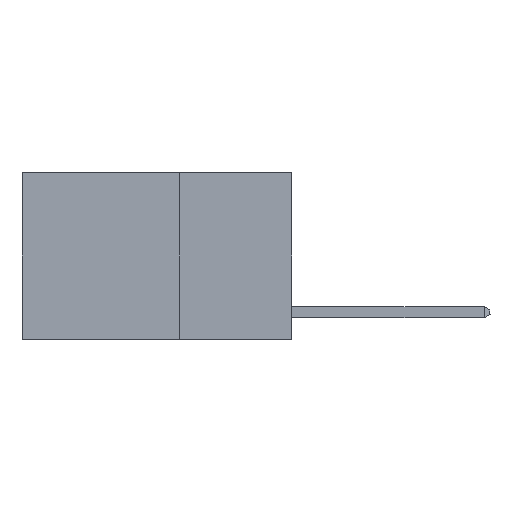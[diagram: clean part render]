
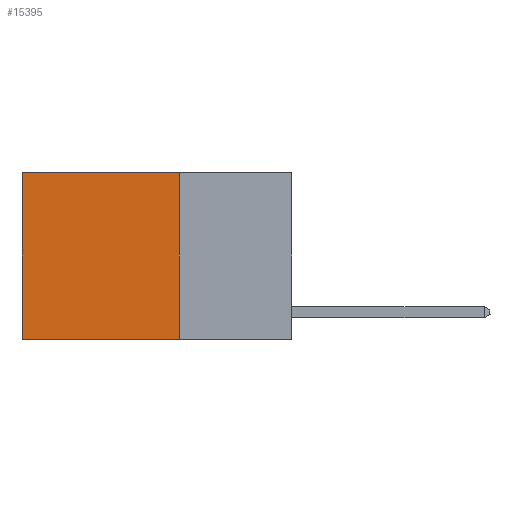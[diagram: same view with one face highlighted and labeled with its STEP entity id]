
A CAD part, left-side view. The second image highlights one B-rep face of the part: STEP entity #15395.
In plain terms, the highlighted planar face has unit normal (-1, 0, 0).
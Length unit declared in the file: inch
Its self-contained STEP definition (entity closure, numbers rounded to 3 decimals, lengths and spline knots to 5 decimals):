
#366 = DIRECTION ( 'NONE',  ( 0., 0., -1. ) ) ;
#754 = ORIENTED_EDGE ( 'NONE', *, *, #4324, .T. ) ;
#1185 = ORIENTED_EDGE ( 'NONE', *, *, #10143, .F. ) ;
#3139 = ORIENTED_EDGE ( 'NONE', *, *, #10969, .F. ) ;
#4324 = EDGE_CURVE ( 'NONE', #18652, #7792, #20906, .T. ) ;
#5500 = DIRECTION ( 'NONE',  ( 0., 1., 0. ) ) ;
#5508 = FACE_OUTER_BOUND ( 'NONE', #6207, .T. ) ;
#5837 = VECTOR ( 'NONE', #5500, 39.37008 ) ;
#6207 = EDGE_LOOP ( 'NONE', ( #754, #1185, #3139, #8943 ) ) ;
#7203 = CARTESIAN_POINT ( 'NONE',  ( 0.2625, 0.25, 0. ) ) ;
#7262 = CARTESIAN_POINT ( 'NONE',  ( 0.2625, 0.25, 0. ) ) ;
#7792 = VERTEX_POINT ( 'NONE', #7804 ) ;
#7804 = CARTESIAN_POINT ( 'NONE',  ( 0.2625, 0.6, -0.37 ) ) ;
#8286 = CARTESIAN_POINT ( 'NONE',  ( 0.2625, 0.25, 0. ) ) ;
#8943 = ORIENTED_EDGE ( 'NONE', *, *, #15745, .T. ) ;
#9602 = CARTESIAN_POINT ( 'NONE',  ( 0.2625, 0.6, 0. ) ) ;
#10048 = DIRECTION ( 'NONE',  ( 0., 0., -1. ) ) ;
#10143 = EDGE_CURVE ( 'NONE', #19412, #7792, #10431, .T. ) ;
#10431 = LINE ( 'NONE', #15563, #5837 ) ;
#10969 = EDGE_CURVE ( 'NONE', #13477, #19412, #16843, .T. ) ;
#12047 = DIRECTION ( 'NONE',  ( 0., 1., 0. ) ) ;
#12719 = VECTOR ( 'NONE', #12984, 39.37008 ) ;
#12984 = DIRECTION ( 'NONE',  ( 0., 0., -1. ) ) ;
#13477 = VERTEX_POINT ( 'NONE', #8286 ) ;
#15219 = LINE ( 'NONE', #15541, #19608 ) ;
#15395 = ADVANCED_FACE ( 'NONE', ( #5508 ), #15571, .F. ) ;
#15541 = CARTESIAN_POINT ( 'NONE',  ( 0.2625, 0.25, 0. ) ) ;
#15563 = CARTESIAN_POINT ( 'NONE',  ( 0.2625, 0.25, -0.37 ) ) ;
#15571 = PLANE ( 'NONE',  #18549 ) ;
#15745 = EDGE_CURVE ( 'NONE', #13477, #18652, #15219, .T. ) ;
#16338 = VECTOR ( 'NONE', #10048, 39.37008 ) ;
#16843 = LINE ( 'NONE', #7203, #16338 ) ;
#17018 = DIRECTION ( 'NONE',  ( 1., 0., 0. ) ) ;
#17111 = CARTESIAN_POINT ( 'NONE',  ( 0.2625, 0.25, -0.37 ) ) ;
#18549 = AXIS2_PLACEMENT_3D ( 'NONE', #7262, #17018, #366 ) ;
#18652 = VERTEX_POINT ( 'NONE', #20900 ) ;
#19412 = VERTEX_POINT ( 'NONE', #17111 ) ;
#19608 = VECTOR ( 'NONE', #12047, 39.37008 ) ;
#20900 = CARTESIAN_POINT ( 'NONE',  ( 0.2625, 0.6, 0. ) ) ;
#20906 = LINE ( 'NONE', #9602, #12719 ) ;
